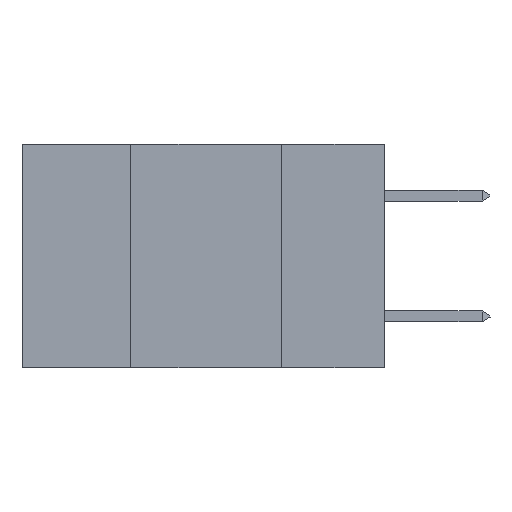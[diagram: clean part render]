
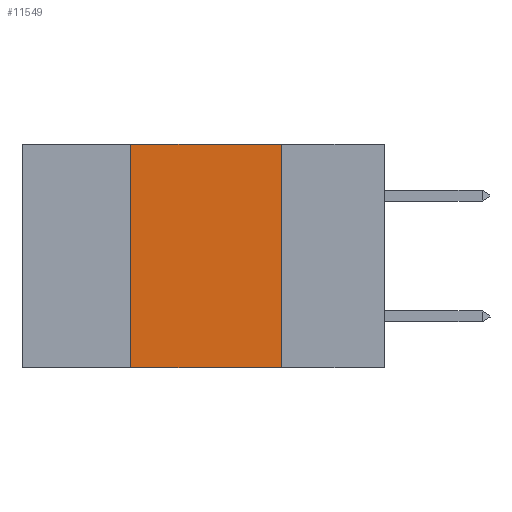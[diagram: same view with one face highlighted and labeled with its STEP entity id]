
A CAD part, left-side view. The second image highlights one B-rep face of the part: STEP entity #11549.
In plain terms, the highlighted planar face has unit normal (-1, 0, 0).
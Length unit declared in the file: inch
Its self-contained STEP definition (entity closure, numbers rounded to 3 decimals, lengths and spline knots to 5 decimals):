
#487 = CARTESIAN_POINT ( 'NONE',  ( 0., 0.17, -0.37 ) ) ;
#2202 = CARTESIAN_POINT ( 'NONE',  ( 0., 0.6, 0. ) ) ;
#2511 = VECTOR ( 'NONE', #22460, 39.37008 ) ;
#3407 = EDGE_CURVE ( 'NONE', #3557, #18073, #24506, .T. ) ;
#3557 = VERTEX_POINT ( 'NONE', #13577 ) ;
#3565 = CARTESIAN_POINT ( 'NONE',  ( 0., 0.6, 0. ) ) ;
#3716 = CARTESIAN_POINT ( 'NONE',  ( 0., 0.17, 0. ) ) ;
#4321 = EDGE_CURVE ( 'NONE', #3557, #9731, #11539, .T. ) ;
#4351 = EDGE_CURVE ( 'NONE', #17984, #18073, #4565, .T. ) ;
#4565 = LINE ( 'NONE', #12168, #7052 ) ;
#4804 = CARTESIAN_POINT ( 'NONE',  ( 0., 0.42, 0. ) ) ;
#5753 = CARTESIAN_POINT ( 'NONE',  ( 0., 0.6, -0.37 ) ) ;
#6573 = DIRECTION ( 'NONE',  ( 0., 0., 1. ) ) ;
#6955 = LINE ( 'NONE', #3565, #2511 ) ;
#7052 = VECTOR ( 'NONE', #19827, 39.37008 ) ;
#9731 = VERTEX_POINT ( 'NONE', #20216 ) ;
#9795 = DIRECTION ( 'NONE',  ( 1., 0., 0. ) ) ;
#10546 = ORIENTED_EDGE ( 'NONE', *, *, #24266, .F. ) ;
#11425 = VECTOR ( 'NONE', #6573, 39.37008 ) ;
#11539 = LINE ( 'NONE', #4804, #11425 ) ;
#11549 = ADVANCED_FACE ( 'NONE', ( #17353 ), #11639, .F. ) ;
#11639 = PLANE ( 'NONE',  #15213 ) ;
#12168 = CARTESIAN_POINT ( 'NONE',  ( 0., 0.17, 0. ) ) ;
#13456 = ORIENTED_EDGE ( 'NONE', *, *, #4321, .F. ) ;
#13577 = CARTESIAN_POINT ( 'NONE',  ( 0., 0.42, -0.37 ) ) ;
#15213 = AXIS2_PLACEMENT_3D ( 'NONE', #2202, #9795, #22942 ) ;
#17353 = FACE_OUTER_BOUND ( 'NONE', #17884, .T. ) ;
#17678 = ORIENTED_EDGE ( 'NONE', *, *, #4351, .F. ) ;
#17884 = EDGE_LOOP ( 'NONE', ( #17678, #10546, #13456, #18323 ) ) ;
#17984 = VERTEX_POINT ( 'NONE', #3716 ) ;
#18073 = VERTEX_POINT ( 'NONE', #487 ) ;
#18323 = ORIENTED_EDGE ( 'NONE', *, *, #3407, .T. ) ;
#18769 = DIRECTION ( 'NONE',  ( 0., -1., 0. ) ) ;
#19827 = DIRECTION ( 'NONE',  ( 0., 0., -1. ) ) ;
#20216 = CARTESIAN_POINT ( 'NONE',  ( 0., 0.42, 0. ) ) ;
#22460 = DIRECTION ( 'NONE',  ( 0., -1., 0. ) ) ;
#22774 = VECTOR ( 'NONE', #18769, 39.37008 ) ;
#22942 = DIRECTION ( 'NONE',  ( 0., 0., -1. ) ) ;
#24266 = EDGE_CURVE ( 'NONE', #9731, #17984, #6955, .T. ) ;
#24506 = LINE ( 'NONE', #5753, #22774 ) ;
